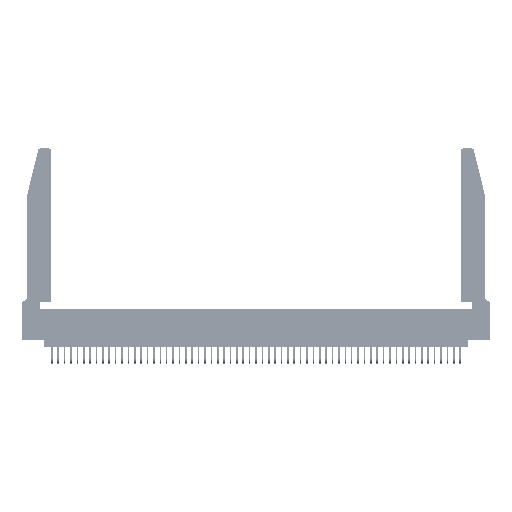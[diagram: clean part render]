
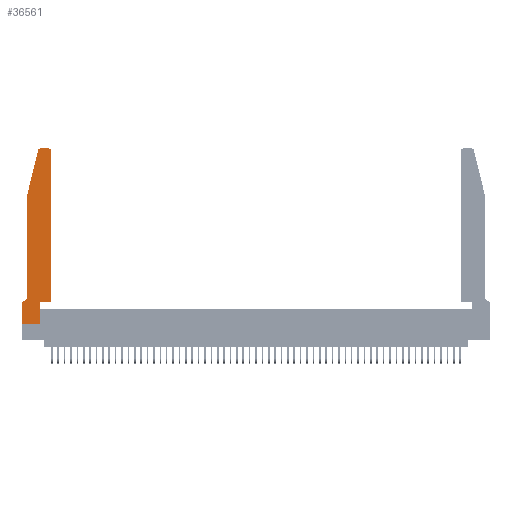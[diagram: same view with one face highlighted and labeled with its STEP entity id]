
A CAD part, top view. The second image highlights one B-rep face of the part: STEP entity #36561.
In plain terms, the highlighted planar face has unit normal (0, 0, 1).
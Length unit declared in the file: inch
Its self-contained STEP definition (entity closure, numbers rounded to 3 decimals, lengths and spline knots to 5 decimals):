
#185 = DIRECTION ( 'NONE',  ( 1., 0., 0. ) ) ;
#415 = LINE ( 'NONE', #52393, #1770 ) ;
#610 = VECTOR ( 'NONE', #5976, 39.37008 ) ;
#1411 = VERTEX_POINT ( 'NONE', #26815 ) ;
#1432 = DIRECTION ( 'NONE',  ( -1., 0., 0. ) ) ;
#1770 = VECTOR ( 'NONE', #23230, 39.37008 ) ;
#2103 = CARTESIAN_POINT ( 'NONE',  ( 0.4505, 2.72, 0.37 ) ) ;
#2273 = VERTEX_POINT ( 'NONE', #33952 ) ;
#2470 = CARTESIAN_POINT ( 'NONE',  ( 0.0055, 0.35, 0.37 ) ) ;
#4517 = CARTESIAN_POINT ( 'NONE',  ( 0.4205, 2.72, 0.37 ) ) ;
#4573 = AXIS2_PLACEMENT_3D ( 'NONE', #8606, #25643, #185 ) ;
#5372 = DIRECTION ( 'NONE',  ( 0., -1., 0. ) ) ;
#5768 = VERTEX_POINT ( 'NONE', #36812 ) ;
#5976 = DIRECTION ( 'NONE',  ( -0.239, -0.971, 0. ) ) ;
#6027 = ORIENTED_EDGE ( 'NONE', *, *, #28281, .T. ) ;
#6612 = EDGE_CURVE ( 'NONE', #40682, #36277, #33802, .T. ) ;
#7443 = ORIENTED_EDGE ( 'NONE', *, *, #43094, .T. ) ;
#8606 = CARTESIAN_POINT ( 'NONE',  ( 0., 0.35, 0.37 ) ) ;
#8750 = VECTOR ( 'NONE', #1432, 39.37008 ) ;
#8807 = DIRECTION ( 'NONE',  ( 1., 0., 0. ) ) ;
#10128 = CARTESIAN_POINT ( 'NONE',  ( 0.284, 2.72, 0.37 ) ) ;
#10377 = CARTESIAN_POINT ( 'NONE',  ( 0.4205, 2.75, 0.37 ) ) ;
#11004 = EDGE_CURVE ( 'NONE', #18699, #23117, #415, .T. ) ;
#12558 = EDGE_CURVE ( 'NONE', #2273, #50757, #49650, .T. ) ;
#13371 = CIRCLE ( 'NONE', #22585, 0.03 ) ;
#13488 = ORIENTED_EDGE ( 'NONE', *, *, #18561, .T. ) ;
#14119 = VECTOR ( 'NONE', #5372, 39.37008 ) ;
#14421 = DIRECTION ( 'NONE',  ( 1., 0., 0. ) ) ;
#14673 = VECTOR ( 'NONE', #49929, 39.37008 ) ;
#15137 = LINE ( 'NONE', #31942, #47326 ) ;
#17207 = DIRECTION ( 'NONE',  ( 0., 0., -1. ) ) ;
#17301 = LINE ( 'NONE', #45738, #14673 ) ;
#17782 = CARTESIAN_POINT ( 'NONE',  ( 0.4505, 0.35, 0.37 ) ) ;
#18561 = EDGE_CURVE ( 'NONE', #45364, #40682, #36518, .T. ) ;
#18624 = CARTESIAN_POINT ( 'NONE',  ( 0.25487, 2.72718, 0.37 ) ) ;
#18699 = VERTEX_POINT ( 'NONE', #10377 ) ;
#19288 = EDGE_CURVE ( 'NONE', #23117, #52564, #13371, .T. ) ;
#19939 = EDGE_CURVE ( 'NONE', #1411, #2273, #47478, .T. ) ;
#21370 = LINE ( 'NONE', #22631, #8750 ) ;
#22585 = AXIS2_PLACEMENT_3D ( 'NONE', #10128, #39576, #14421 ) ;
#22631 = CARTESIAN_POINT ( 'NONE',  ( 0.0755, 0.35, 0.37 ) ) ;
#23117 = VERTEX_POINT ( 'NONE', #30653 ) ;
#23230 = DIRECTION ( 'NONE',  ( -1., 0., 0. ) ) ;
#23819 = CARTESIAN_POINT ( 'NONE',  ( 0.4505, 0.35, 0.37 ) ) ;
#24032 = ORIENTED_EDGE ( 'NONE', *, *, #11004, .T. ) ;
#24423 = ORIENTED_EDGE ( 'NONE', *, *, #51896, .T. ) ;
#25217 = VECTOR ( 'NONE', #28046, 39.37008 ) ;
#25219 = VECTOR ( 'NONE', #41464, 39.37008 ) ;
#25643 = DIRECTION ( 'NONE',  ( 0., 0., 1. ) ) ;
#26815 = CARTESIAN_POINT ( 'NONE',  ( 0.2865, 0.35, 0.37 ) ) ;
#27190 = ORIENTED_EDGE ( 'NONE', *, *, #52986, .T. ) ;
#28046 = DIRECTION ( 'NONE',  ( 1., 0., 0. ) ) ;
#28205 = CARTESIAN_POINT ( 'NONE',  ( 0., 0.35, 0.37 ) ) ;
#28281 = EDGE_CURVE ( 'NONE', #51298, #5768, #17301, .T. ) ;
#28662 = ORIENTED_EDGE ( 'NONE', *, *, #46594, .T. ) ;
#28762 = VERTEX_POINT ( 'NONE', #28205 ) ;
#29803 = ORIENTED_EDGE ( 'NONE', *, *, #19288, .T. ) ;
#30653 = CARTESIAN_POINT ( 'NONE',  ( 0.284, 2.75, 0.37 ) ) ;
#30692 = CIRCLE ( 'NONE', #47585, 0.03 ) ;
#30745 = CARTESIAN_POINT ( 'NONE',  ( 0.0755, 2., 0.37 ) ) ;
#31699 = ORIENTED_EDGE ( 'NONE', *, *, #6612, .T. ) ;
#31942 = CARTESIAN_POINT ( 'NONE',  ( 0., 0., 0.37 ) ) ;
#33802 = CIRCLE ( 'NONE', #38519, 0.07 ) ;
#33952 = CARTESIAN_POINT ( 'NONE',  ( 0.4505, 0.35, 0.37 ) ) ;
#34103 = DIRECTION ( 'NONE',  ( 0., 0., 1. ) ) ;
#34849 = EDGE_CURVE ( 'NONE', #5768, #1411, #48748, .T. ) ;
#35407 = ORIENTED_EDGE ( 'NONE', *, *, #34849, .T. ) ;
#35535 = CARTESIAN_POINT ( 'NONE',  ( 0.0755, 2., 0.37 ) ) ;
#36277 = VERTEX_POINT ( 'NONE', #2470 ) ;
#36405 = FACE_OUTER_BOUND ( 'NONE', #50861, .T. ) ;
#36518 = LINE ( 'NONE', #30745, #14119 ) ;
#36561 = ADVANCED_FACE ( 'NONE', ( #36405 ), #50627, .T. ) ;
#36812 = CARTESIAN_POINT ( 'NONE',  ( 0.2865, 0., 0.37 ) ) ;
#38519 = AXIS2_PLACEMENT_3D ( 'NONE', #42331, #17207, #46582 ) ;
#39314 = CARTESIAN_POINT ( 'NONE',  ( 0., 0., 0.37 ) ) ;
#39576 = DIRECTION ( 'NONE',  ( 0., 0., 1. ) ) ;
#40682 = VERTEX_POINT ( 'NONE', #40945 ) ;
#40945 = CARTESIAN_POINT ( 'NONE',  ( 0.0755, 0.42, 0.37 ) ) ;
#41464 = DIRECTION ( 'NONE',  ( 0., 1., 0. ) ) ;
#42331 = CARTESIAN_POINT ( 'NONE',  ( 0.0055, 0.42, 0.37 ) ) ;
#42893 = DIRECTION ( 'NONE',  ( 0., 1., 0. ) ) ;
#43094 = EDGE_CURVE ( 'NONE', #28762, #51298, #15137, .T. ) ;
#44497 = DIRECTION ( 'NONE',  ( 0., -1., 0. ) ) ;
#45364 = VERTEX_POINT ( 'NONE', #46798 ) ;
#45456 = LINE ( 'NONE', #35535, #610 ) ;
#45662 = CARTESIAN_POINT ( 'NONE',  ( 0.2865, 0.35, 0.37 ) ) ;
#45738 = CARTESIAN_POINT ( 'NONE',  ( 0., 0., 0.37 ) ) ;
#46582 = DIRECTION ( 'NONE',  ( -1., 0., 0. ) ) ;
#46594 = EDGE_CURVE ( 'NONE', #50757, #18699, #30692, .T. ) ;
#46798 = CARTESIAN_POINT ( 'NONE',  ( 0.0755, 2., 0.37 ) ) ;
#47088 = VECTOR ( 'NONE', #42893, 39.37008 ) ;
#47294 = ORIENTED_EDGE ( 'NONE', *, *, #19939, .T. ) ;
#47326 = VECTOR ( 'NONE', #44497, 39.37008 ) ;
#47478 = LINE ( 'NONE', #23819, #25217 ) ;
#47585 = AXIS2_PLACEMENT_3D ( 'NONE', #4517, #34103, #8807 ) ;
#47818 = ORIENTED_EDGE ( 'NONE', *, *, #12558, .T. ) ;
#48748 = LINE ( 'NONE', #45662, #25219 ) ;
#49650 = LINE ( 'NONE', #17782, #47088 ) ;
#49929 = DIRECTION ( 'NONE',  ( 1., 0., 0. ) ) ;
#50627 = PLANE ( 'NONE',  #4573 ) ;
#50757 = VERTEX_POINT ( 'NONE', #2103 ) ;
#50861 = EDGE_LOOP ( 'NONE', ( #24032, #29803, #27190, #13488, #31699, #24423, #7443, #6027, #35407, #47294, #47818, #28662 ) ) ;
#51298 = VERTEX_POINT ( 'NONE', #39314 ) ;
#51896 = EDGE_CURVE ( 'NONE', #36277, #28762, #21370, .T. ) ;
#52393 = CARTESIAN_POINT ( 'NONE',  ( 0.2605, 2.75, 0.37 ) ) ;
#52564 = VERTEX_POINT ( 'NONE', #18624 ) ;
#52986 = EDGE_CURVE ( 'NONE', #52564, #45364, #45456, .T. ) ;
